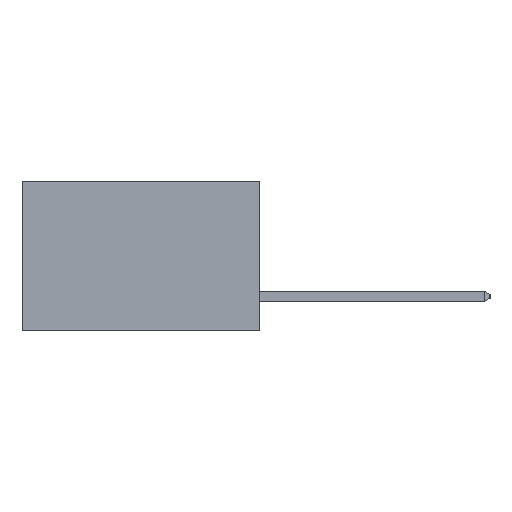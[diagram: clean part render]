
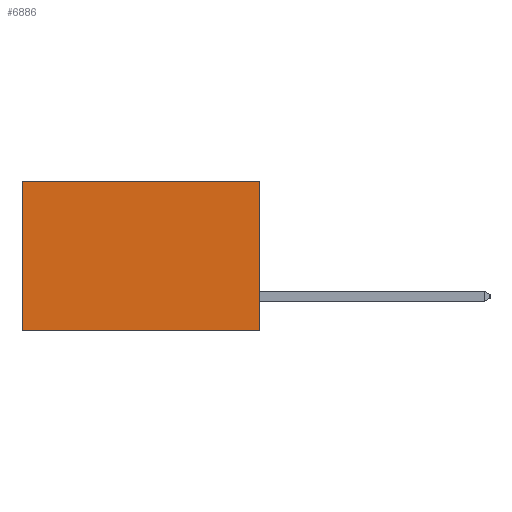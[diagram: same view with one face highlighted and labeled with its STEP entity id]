
A CAD part, left-side view. The second image highlights one B-rep face of the part: STEP entity #6886.
In plain terms, the highlighted planar face has unit normal (-1, 0, 0).
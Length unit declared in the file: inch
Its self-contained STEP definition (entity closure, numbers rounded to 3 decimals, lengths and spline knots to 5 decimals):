
#505 = EDGE_CURVE ( 'NONE', #5953, #9884, #6985, .T. ) ;
#758 = ORIENTED_EDGE ( 'NONE', *, *, #9097, .T. ) ;
#814 = ORIENTED_EDGE ( 'NONE', *, *, #11737, .F. ) ;
#1583 = VECTOR ( 'NONE', #3952, 39.37008 ) ;
#1854 = CARTESIAN_POINT ( 'NONE',  ( 0.277, 0., 0. ) ) ;
#1933 = LINE ( 'NONE', #2878, #1583 ) ;
#2364 = DIRECTION ( 'NONE',  ( 0., 0., -1. ) ) ;
#2367 = DIRECTION ( 'NONE',  ( 1., 0., 0. ) ) ;
#2397 = CARTESIAN_POINT ( 'NONE',  ( 0.277, 0., -0.37 ) ) ;
#2493 = PLANE ( 'NONE',  #8267 ) ;
#2878 = CARTESIAN_POINT ( 'NONE',  ( 0.277, 0., -0.37 ) ) ;
#3164 = CARTESIAN_POINT ( 'NONE',  ( 0.277, 0.59, 0. ) ) ;
#3667 = ORIENTED_EDGE ( 'NONE', *, *, #11338, .F. ) ;
#3851 = LINE ( 'NONE', #1854, #11551 ) ;
#3952 = DIRECTION ( 'NONE',  ( 0., 1., 0. ) ) ;
#4472 = LINE ( 'NONE', #13061, #12094 ) ;
#5405 = VERTEX_POINT ( 'NONE', #6709 ) ;
#5953 = VERTEX_POINT ( 'NONE', #3164 ) ;
#6709 = CARTESIAN_POINT ( 'NONE',  ( 0.277, 0., -0.37 ) ) ;
#6886 = ADVANCED_FACE ( 'NONE', ( #7248 ), #2493, .F. ) ;
#6985 = LINE ( 'NONE', #9696, #9335 ) ;
#7248 = FACE_OUTER_BOUND ( 'NONE', #10960, .T. ) ;
#8248 = ORIENTED_EDGE ( 'NONE', *, *, #505, .T. ) ;
#8267 = AXIS2_PLACEMENT_3D ( 'NONE', #2397, #2367, #2364 ) ;
#8321 = CARTESIAN_POINT ( 'NONE',  ( 0.277, 0., 0. ) ) ;
#9097 = EDGE_CURVE ( 'NONE', #9259, #5953, #3851, .T. ) ;
#9259 = VERTEX_POINT ( 'NONE', #8321 ) ;
#9335 = VECTOR ( 'NONE', #11452, 39.37008 ) ;
#9452 = CARTESIAN_POINT ( 'NONE',  ( 0.277, 0.59, -0.37 ) ) ;
#9696 = CARTESIAN_POINT ( 'NONE',  ( 0.277, 0.59, -0.37 ) ) ;
#9884 = VERTEX_POINT ( 'NONE', #9452 ) ;
#10059 = DIRECTION ( 'NONE',  ( 0., 1., 0. ) ) ;
#10128 = DIRECTION ( 'NONE',  ( 0., 0., -1. ) ) ;
#10960 = EDGE_LOOP ( 'NONE', ( #8248, #814, #3667, #758 ) ) ;
#11338 = EDGE_CURVE ( 'NONE', #9259, #5405, #4472, .T. ) ;
#11452 = DIRECTION ( 'NONE',  ( 0., 0., -1. ) ) ;
#11551 = VECTOR ( 'NONE', #10059, 39.37008 ) ;
#11737 = EDGE_CURVE ( 'NONE', #5405, #9884, #1933, .T. ) ;
#12094 = VECTOR ( 'NONE', #10128, 39.37008 ) ;
#13061 = CARTESIAN_POINT ( 'NONE',  ( 0.277, 0., -0.37 ) ) ;
